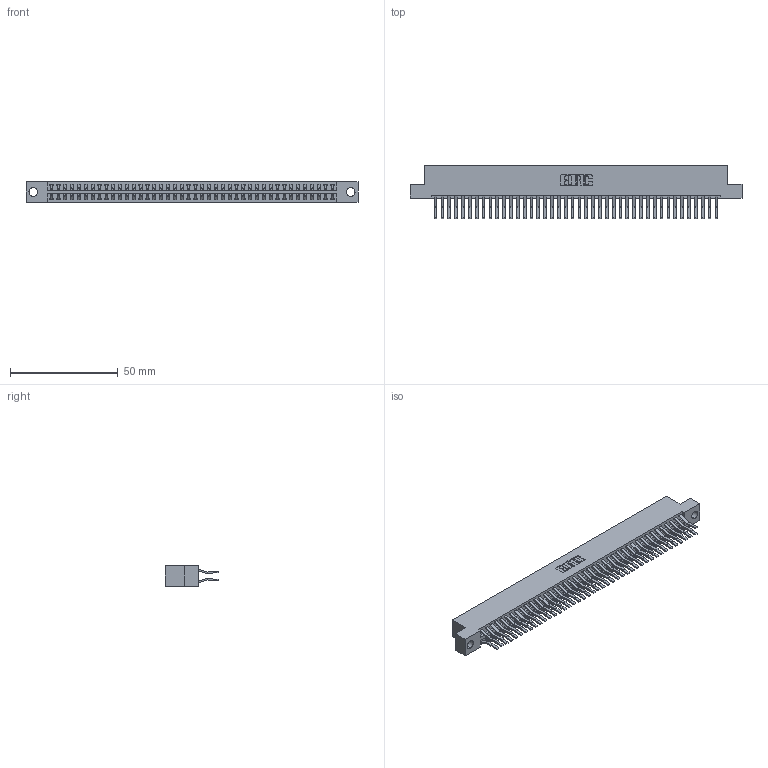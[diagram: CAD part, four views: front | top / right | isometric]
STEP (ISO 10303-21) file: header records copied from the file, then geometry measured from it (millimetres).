
FILE_DESCRIPTION (( 'STEP AP203' ), '1' );
FILE_NAME ('346-084-560-204.STEP', '2022-05-25T21:14:22', ( '' ), ( '' ), 'SwSTEP 2.0', 'SolidWorks 2020', '' );
FILE_SCHEMA (( 'CONFIG_CONTROL_DESIGN' ));
Length unit declared in the file: inch
Products named in the file (3): 345-292-001_560 Tail; 346-084-560-204; 346 Part_Flush Mounting Lugs - 0.156 Dia-TH
Assembly tree (85 placements, depth 2):
  346-084-560-204
    346 Part_Flush Mounting Lugs - 0.156 Dia-TH
    345-292-001_560 Tail  x84
Bounding box: 153.92 x 24.78 x 9.4 mm (x, y, z)
Volume: 15454.1 mm3; surface area: 22559.6 mm2
Topology: 85 solids, 85 shells, 4672 faces, 13889 edges, 9146 vertices
Faces by surface type: plane 3030, cylinder 1642
Entity records: 27917 total; most frequent: CARTESIAN_POINT 4606, ORIENTED_EDGE 4538, DIRECTION 4113, EDGE_CURVE 2269, LINE 1965, VECTOR 1965, VERTEX_POINT 1510, AXIS2_PLACEMENT_3D 1074
